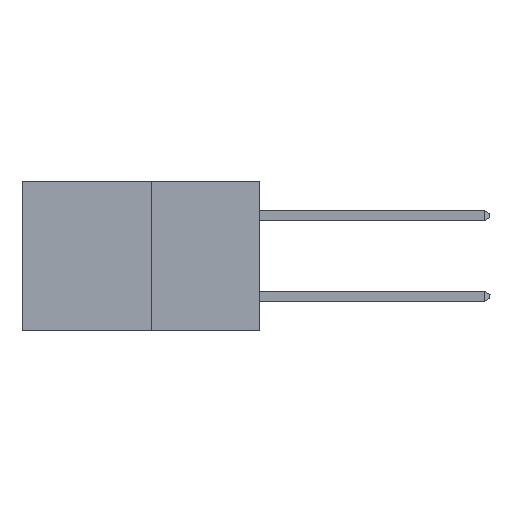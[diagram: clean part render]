
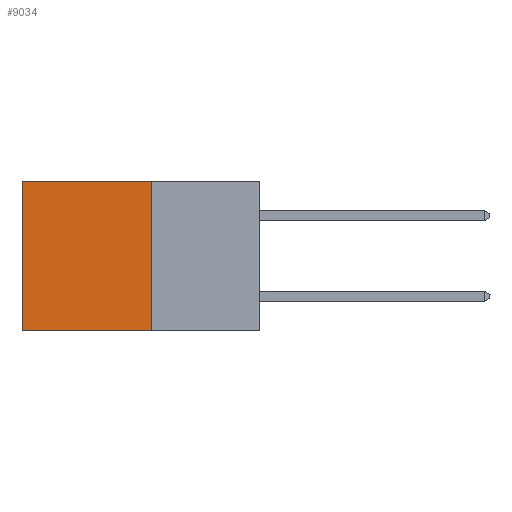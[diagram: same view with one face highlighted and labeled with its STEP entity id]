
A CAD part, left-side view. The second image highlights one B-rep face of the part: STEP entity #9034.
In plain terms, the highlighted planar face has unit normal (-1, 0, 0).
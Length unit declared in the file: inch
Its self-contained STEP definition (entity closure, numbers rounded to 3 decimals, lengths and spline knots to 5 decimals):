
#579 = EDGE_CURVE ( 'NONE', #6314, #7130, #3871, .T. ) ;
#1350 = EDGE_CURVE ( 'NONE', #11194, #6314, #7349, .T. ) ;
#1921 = VECTOR ( 'NONE', #4685, 39.37008 ) ;
#2250 = ORIENTED_EDGE ( 'NONE', *, *, #579, .F. ) ;
#3613 = ORIENTED_EDGE ( 'NONE', *, *, #10615, .T. ) ;
#3871 = LINE ( 'NONE', #5784, #8294 ) ;
#4083 = DIRECTION ( 'NONE',  ( 0., 0., -1. ) ) ;
#4257 = DIRECTION ( 'NONE',  ( 0., 1., 0. ) ) ;
#4321 = CARTESIAN_POINT ( 'NONE',  ( 0.277, 0.27, -0.37 ) ) ;
#4338 = CARTESIAN_POINT ( 'NONE',  ( 0.277, 0.27, -0.37 ) ) ;
#4390 = CARTESIAN_POINT ( 'NONE',  ( 0.277, 0.27, -0.37 ) ) ;
#4535 = AXIS2_PLACEMENT_3D ( 'NONE', #4338, #11160, #6175 ) ;
#4685 = DIRECTION ( 'NONE',  ( 0., 0., -1. ) ) ;
#4702 = CARTESIAN_POINT ( 'NONE',  ( 0.277, 0.59, -0.37 ) ) ;
#4966 = CARTESIAN_POINT ( 'NONE',  ( 0.277, 0.59, 0. ) ) ;
#5131 = EDGE_CURVE ( 'NONE', #6777, #7130, #7029, .T. ) ;
#5272 = PLANE ( 'NONE',  #4535 ) ;
#5353 = FACE_OUTER_BOUND ( 'NONE', #9647, .T. ) ;
#5784 = CARTESIAN_POINT ( 'NONE',  ( 0.277, 0.27, -0.37 ) ) ;
#5998 = DIRECTION ( 'NONE',  ( 0., 1., 0. ) ) ;
#6175 = DIRECTION ( 'NONE',  ( 0., 0., -1. ) ) ;
#6314 = VERTEX_POINT ( 'NONE', #4390 ) ;
#6340 = ORIENTED_EDGE ( 'NONE', *, *, #1350, .F. ) ;
#6777 = VERTEX_POINT ( 'NONE', #4966 ) ;
#7029 = LINE ( 'NONE', #4702, #1921 ) ;
#7130 = VERTEX_POINT ( 'NONE', #11260 ) ;
#7349 = LINE ( 'NONE', #4321, #11460 ) ;
#7576 = CARTESIAN_POINT ( 'NONE',  ( 0.277, 0.27, 0. ) ) ;
#7782 = CARTESIAN_POINT ( 'NONE',  ( 0.277, 0.27, 0. ) ) ;
#8294 = VECTOR ( 'NONE', #5998, 39.37008 ) ;
#8693 = LINE ( 'NONE', #7782, #8948 ) ;
#8948 = VECTOR ( 'NONE', #4257, 39.37008 ) ;
#9034 = ADVANCED_FACE ( 'NONE', ( #5353 ), #5272, .F. ) ;
#9647 = EDGE_LOOP ( 'NONE', ( #10665, #2250, #6340, #3613 ) ) ;
#10615 = EDGE_CURVE ( 'NONE', #11194, #6777, #8693, .T. ) ;
#10665 = ORIENTED_EDGE ( 'NONE', *, *, #5131, .T. ) ;
#11160 = DIRECTION ( 'NONE',  ( 1., 0., 0. ) ) ;
#11194 = VERTEX_POINT ( 'NONE', #7576 ) ;
#11260 = CARTESIAN_POINT ( 'NONE',  ( 0.277, 0.59, -0.37 ) ) ;
#11460 = VECTOR ( 'NONE', #4083, 39.37008 ) ;
